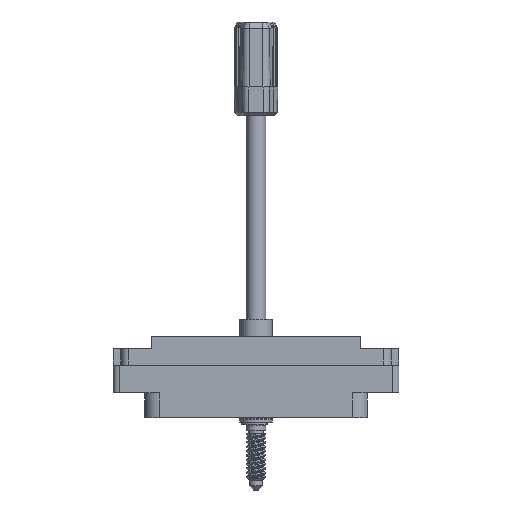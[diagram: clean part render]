
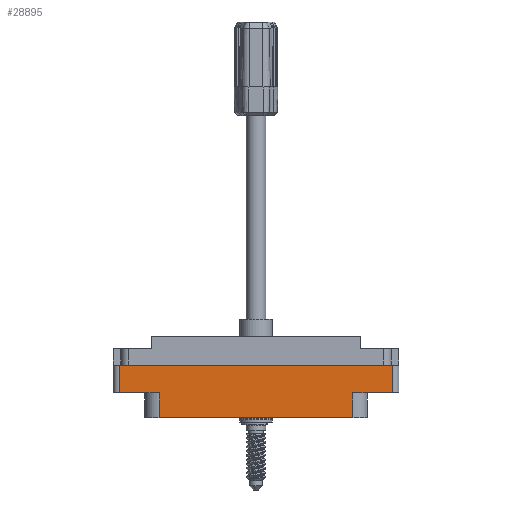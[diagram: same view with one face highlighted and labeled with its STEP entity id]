
A CAD part, front view. The second image highlights one B-rep face of the part: STEP entity #28895.
In plain terms, the highlighted planar face has unit normal (0, -1, 0).
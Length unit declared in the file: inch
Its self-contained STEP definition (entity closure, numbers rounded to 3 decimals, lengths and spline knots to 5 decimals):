
#646 = CARTESIAN_POINT ( 'NONE',  ( 0., -0.7625, -0.54 ) ) ;
#2559 = VECTOR ( 'NONE', #27014, 39.37008 ) ;
#2849 = LINE ( 'NONE', #646, #19256 ) ;
#3757 = LINE ( 'NONE', #71775, #2559 ) ;
#8812 = DIRECTION ( 'NONE',  ( -1., 0., 0. ) ) ;
#9854 = CARTESIAN_POINT ( 'NONE',  ( -0.9315, -0.7625, -0.78 ) ) ;
#11596 = CARTESIAN_POINT ( 'NONE',  ( -1.313, -0.7625, -0.54 ) ) ;
#12323 = CARTESIAN_POINT ( 'NONE',  ( 0.9315, -0.7625, -0.54 ) ) ;
#14376 = VERTEX_POINT ( 'NONE', #11596 ) ;
#16183 = VERTEX_POINT ( 'NONE', #9854 ) ;
#17198 = ORIENTED_EDGE ( 'NONE', *, *, #43595, .T. ) ;
#17378 = VERTEX_POINT ( 'NONE', #47547 ) ;
#19256 = VECTOR ( 'NONE', #8812, 39.37008 ) ;
#19845 = CARTESIAN_POINT ( 'NONE',  ( 0., -0.7625, -0.54 ) ) ;
#23401 = CARTESIAN_POINT ( 'NONE',  ( 0.9315, -0.7625, -0.54 ) ) ;
#24492 = LINE ( 'NONE', #19845, #57172 ) ;
#26427 = DIRECTION ( 'NONE',  ( 1., 0., 0. ) ) ;
#27014 = DIRECTION ( 'NONE',  ( 1., 0., 0. ) ) ;
#28895 = ADVANCED_FACE ( 'NONE', ( #55408 ), #32758, .T. ) ;
#32758 = PLANE ( 'NONE',  #42917 ) ;
#33588 = ORIENTED_EDGE ( 'NONE', *, *, #64443, .T. ) ;
#35811 = ORIENTED_EDGE ( 'NONE', *, *, #61730, .F. ) ;
#36680 = LINE ( 'NONE', #23401, #74048 ) ;
#36857 = ORIENTED_EDGE ( 'NONE', *, *, #75947, .T. ) ;
#38075 = DIRECTION ( 'NONE',  ( 0., 0., 1. ) ) ;
#40256 = VERTEX_POINT ( 'NONE', #74161 ) ;
#42121 = CARTESIAN_POINT ( 'NONE',  ( 0., -0.7625, -0.274 ) ) ;
#42917 = AXIS2_PLACEMENT_3D ( 'NONE', #55942, #71296, #78152 ) ;
#42967 = CARTESIAN_POINT ( 'NONE',  ( 1.313, -0.7625, -0.274 ) ) ;
#43595 = EDGE_CURVE ( 'NONE', #17378, #16183, #78277, .T. ) ;
#45379 = ORIENTED_EDGE ( 'NONE', *, *, #62310, .T. ) ;
#47547 = CARTESIAN_POINT ( 'NONE',  ( -0.9315, -0.7625, -0.54 ) ) ;
#50185 = VECTOR ( 'NONE', #26427, 39.37008 ) ;
#51009 = EDGE_CURVE ( 'NONE', #16183, #40256, #3757, .T. ) ;
#51980 = VERTEX_POINT ( 'NONE', #42967 ) ;
#55408 = FACE_OUTER_BOUND ( 'NONE', #78790, .T. ) ;
#55942 = CARTESIAN_POINT ( 'NONE',  ( -1.375, -0.7625, -0.78 ) ) ;
#56059 = VECTOR ( 'NONE', #96834, 39.37008 ) ;
#57172 = VECTOR ( 'NONE', #72086, 39.37008 ) ;
#61730 = EDGE_CURVE ( 'NONE', #76543, #77294, #2849, .T. ) ;
#61985 = VECTOR ( 'NONE', #71697, 39.37008 ) ;
#62310 = EDGE_CURVE ( 'NONE', #40256, #77294, #36680, .T. ) ;
#64443 = EDGE_CURVE ( 'NONE', #76543, #51980, #73575, .T. ) ;
#64750 = EDGE_CURVE ( 'NONE', #87393, #51980, #70067, .T. ) ;
#68995 = CARTESIAN_POINT ( 'NONE',  ( -1.313, -0.7625, -0.274 ) ) ;
#70067 = LINE ( 'NONE', #42121, #50185 ) ;
#71296 = DIRECTION ( 'NONE',  ( 0., -1., 0. ) ) ;
#71697 = DIRECTION ( 'NONE',  ( 0., 0., 1. ) ) ;
#71775 = CARTESIAN_POINT ( 'NONE',  ( -1.375, -0.7625, -0.78 ) ) ;
#72086 = DIRECTION ( 'NONE',  ( 1., 0., 0. ) ) ;
#73575 = LINE ( 'NONE', #92656, #61985 ) ;
#74048 = VECTOR ( 'NONE', #38075, 39.37008 ) ;
#74161 = CARTESIAN_POINT ( 'NONE',  ( 0.9315, -0.7625, -0.78 ) ) ;
#75947 = EDGE_CURVE ( 'NONE', #14376, #17378, #24492, .T. ) ;
#76543 = VERTEX_POINT ( 'NONE', #95827 ) ;
#77294 = VERTEX_POINT ( 'NONE', #12323 ) ;
#78152 = DIRECTION ( 'NONE',  ( 0., 0., -1. ) ) ;
#78277 = LINE ( 'NONE', #96520, #56059 ) ;
#78283 = VECTOR ( 'NONE', #95207, 39.37008 ) ;
#78790 = EDGE_LOOP ( 'NONE', ( #94595, #95379, #36857, #17198, #95360, #45379, #35811, #33588 ) ) ;
#84494 = EDGE_CURVE ( 'NONE', #87393, #14376, #85303, .T. ) ;
#85303 = LINE ( 'NONE', #87678, #78283 ) ;
#87393 = VERTEX_POINT ( 'NONE', #68995 ) ;
#87678 = CARTESIAN_POINT ( 'NONE',  ( -1.313, -0.7625, -0.78 ) ) ;
#92656 = CARTESIAN_POINT ( 'NONE',  ( 1.313, -0.7625, -0.78 ) ) ;
#94595 = ORIENTED_EDGE ( 'NONE', *, *, #64750, .F. ) ;
#95207 = DIRECTION ( 'NONE',  ( 0., 0., -1. ) ) ;
#95360 = ORIENTED_EDGE ( 'NONE', *, *, #51009, .T. ) ;
#95379 = ORIENTED_EDGE ( 'NONE', *, *, #84494, .T. ) ;
#95827 = CARTESIAN_POINT ( 'NONE',  ( 1.313, -0.7625, -0.54 ) ) ;
#96520 = CARTESIAN_POINT ( 'NONE',  ( -0.9315, -0.7625, -0.78 ) ) ;
#96834 = DIRECTION ( 'NONE',  ( 0., 0., -1. ) ) ;
